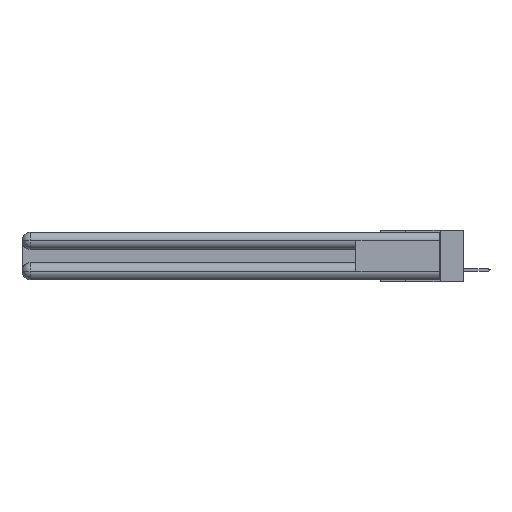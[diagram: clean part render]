
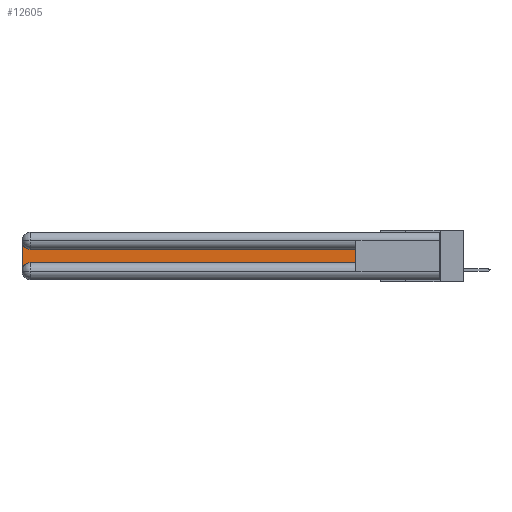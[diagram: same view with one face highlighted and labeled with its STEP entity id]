
A CAD part, left-side view. The second image highlights one B-rep face of the part: STEP entity #12605.
In plain terms, the highlighted planar face has unit normal (-1, 0, 0).
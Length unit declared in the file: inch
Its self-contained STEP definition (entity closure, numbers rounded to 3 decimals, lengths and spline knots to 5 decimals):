
#1459 = CIRCLE ( 'NONE', #6020, 0.06 ) ;
#2593 = ORIENTED_EDGE ( 'NONE', *, *, #8842, .T. ) ;
#2837 = VECTOR ( 'NONE', #15058, 39.37008 ) ;
#3675 = DIRECTION ( 'NONE',  ( 1., 0., 0. ) ) ;
#4466 = VERTEX_POINT ( 'NONE', #10602 ) ;
#4703 = ORIENTED_EDGE ( 'NONE', *, *, #26129, .T. ) ;
#4755 = LINE ( 'NONE', #11653, #9934 ) ;
#5216 = CARTESIAN_POINT ( 'NONE',  ( 0.075, 2.94, -0.1225 ) ) ;
#5973 = CARTESIAN_POINT ( 'NONE',  ( 0.075, 3., -0.1225 ) ) ;
#6020 = AXIS2_PLACEMENT_3D ( 'NONE', #23641, #28079, #10414 ) ;
#6434 = AXIS2_PLACEMENT_3D ( 'NONE', #5973, #10731, #8568 ) ;
#7244 = AXIS2_PLACEMENT_3D ( 'NONE', #28004, #3675, #8475 ) ;
#7246 = EDGE_CURVE ( 'NONE', #18144, #10926, #27989, .T. ) ;
#7878 = VERTEX_POINT ( 'NONE', #16190 ) ;
#8318 = CARTESIAN_POINT ( 'NONE',  ( 0.075, 3., -0.0625 ) ) ;
#8475 = DIRECTION ( 'NONE',  ( 0., 0., -1. ) ) ;
#8561 = CARTESIAN_POINT ( 'NONE',  ( 0.075, 0.6, -0.1225 ) ) ;
#8568 = DIRECTION ( 'NONE',  ( 0., 0., -1. ) ) ;
#8656 = EDGE_CURVE ( 'NONE', #20828, #4466, #1459, .T. ) ;
#8842 = EDGE_CURVE ( 'NONE', #4466, #7878, #23919, .T. ) ;
#9934 = VECTOR ( 'NONE', #13683, 39.37008 ) ;
#9951 = ORIENTED_EDGE ( 'NONE', *, *, #8656, .T. ) ;
#10414 = DIRECTION ( 'NONE',  ( 0., 0., -1. ) ) ;
#10602 = CARTESIAN_POINT ( 'NONE',  ( 0.075, 2.94, -0.2175 ) ) ;
#10731 = DIRECTION ( 'NONE',  ( 1., 0., 0. ) ) ;
#10926 = VERTEX_POINT ( 'NONE', #8318 ) ;
#11653 = CARTESIAN_POINT ( 'NONE',  ( 0.075, 3., -0.2175 ) ) ;
#12605 = ADVANCED_FACE ( 'NONE', ( #13025 ), #23749, .F. ) ;
#12785 = DIRECTION ( 'NONE',  ( 0., -1., 0. ) ) ;
#13025 = FACE_OUTER_BOUND ( 'NONE', #28559, .T. ) ;
#13448 = CARTESIAN_POINT ( 'NONE',  ( 0.075, 3., -0.2775 ) ) ;
#13615 = ORIENTED_EDGE ( 'NONE', *, *, #28490, .T. ) ;
#13683 = DIRECTION ( 'NONE',  ( 0., 0., -1. ) ) ;
#13803 = VECTOR ( 'NONE', #14678, 39.37008 ) ;
#14678 = DIRECTION ( 'NONE',  ( 0., 0., 1. ) ) ;
#15058 = DIRECTION ( 'NONE',  ( 0., 1., 0. ) ) ;
#16190 = CARTESIAN_POINT ( 'NONE',  ( 0.075, 0.6, -0.2175 ) ) ;
#16736 = CARTESIAN_POINT ( 'NONE',  ( 0.075, 0.6, -0.1225 ) ) ;
#18144 = VERTEX_POINT ( 'NONE', #5216 ) ;
#18295 = LINE ( 'NONE', #23264, #13803 ) ;
#19650 = VERTEX_POINT ( 'NONE', #16736 ) ;
#20451 = VECTOR ( 'NONE', #12785, 39.37008 ) ;
#20828 = VERTEX_POINT ( 'NONE', #13448 ) ;
#20831 = LINE ( 'NONE', #8561, #2837 ) ;
#22890 = EDGE_CURVE ( 'NONE', #10926, #20828, #4755, .T. ) ;
#23264 = CARTESIAN_POINT ( 'NONE',  ( 0.075, 0.6, -0.2175 ) ) ;
#23641 = CARTESIAN_POINT ( 'NONE',  ( 0.075, 2.94, -0.2775 ) ) ;
#23749 = PLANE ( 'NONE',  #6434 ) ;
#23919 = LINE ( 'NONE', #28318, #20451 ) ;
#25716 = ORIENTED_EDGE ( 'NONE', *, *, #7246, .T. ) ;
#26129 = EDGE_CURVE ( 'NONE', #19650, #18144, #20831, .T. ) ;
#27989 = CIRCLE ( 'NONE', #7244, 0.06 ) ;
#28004 = CARTESIAN_POINT ( 'NONE',  ( 0.075, 2.94, -0.0625 ) ) ;
#28079 = DIRECTION ( 'NONE',  ( 1., 0., 0. ) ) ;
#28181 = ORIENTED_EDGE ( 'NONE', *, *, #22890, .T. ) ;
#28318 = CARTESIAN_POINT ( 'NONE',  ( 0.075, 0.6, -0.2175 ) ) ;
#28490 = EDGE_CURVE ( 'NONE', #7878, #19650, #18295, .T. ) ;
#28559 = EDGE_LOOP ( 'NONE', ( #4703, #25716, #28181, #9951, #2593, #13615 ) ) ;
